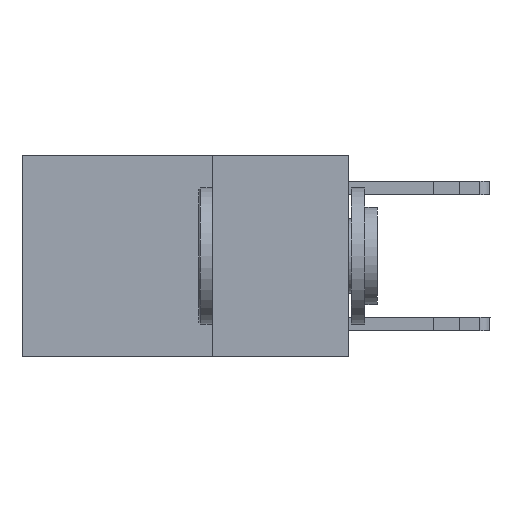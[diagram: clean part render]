
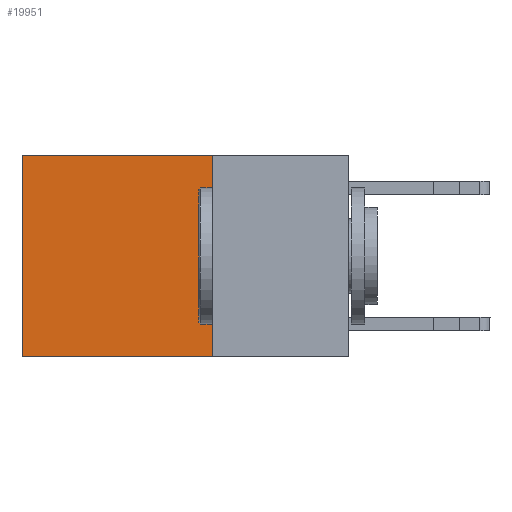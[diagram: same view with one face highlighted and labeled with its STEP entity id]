
A CAD part, left-side view. The second image highlights one B-rep face of the part: STEP entity #19951.
In plain terms, the highlighted planar face has unit normal (-1, 0, 0).
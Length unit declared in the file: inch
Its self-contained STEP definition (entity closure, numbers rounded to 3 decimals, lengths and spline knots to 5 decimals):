
#849 = VERTEX_POINT ( 'NONE', #15176 ) ;
#2041 = VERTEX_POINT ( 'NONE', #2257 ) ;
#2257 = CARTESIAN_POINT ( 'NONE',  ( 0.2625, 0.25, -0.37 ) ) ;
#2558 = EDGE_LOOP ( 'NONE', ( #5270, #16723, #10378, #8038 ) ) ;
#3212 = DIRECTION ( 'NONE',  ( 0., 0., -1. ) ) ;
#3309 = DIRECTION ( 'NONE',  ( 1., 0., 0. ) ) ;
#3355 = CARTESIAN_POINT ( 'NONE',  ( 0.2625, 0.25, 0. ) ) ;
#4119 = PLANE ( 'NONE',  #19130 ) ;
#4580 = EDGE_CURVE ( 'NONE', #13474, #21646, #9042, .T. ) ;
#5270 = ORIENTED_EDGE ( 'NONE', *, *, #4580, .T. ) ;
#5322 = CARTESIAN_POINT ( 'NONE',  ( 0.2625, 0.6, -0.37 ) ) ;
#5961 = CARTESIAN_POINT ( 'NONE',  ( 0.2625, 0.6, 0. ) ) ;
#8038 = ORIENTED_EDGE ( 'NONE', *, *, #8169, .T. ) ;
#8169 = EDGE_CURVE ( 'NONE', #849, #13474, #14391, .T. ) ;
#8604 = VECTOR ( 'NONE', #12992, 39.37008 ) ;
#9042 = LINE ( 'NONE', #13243, #8604 ) ;
#10378 = ORIENTED_EDGE ( 'NONE', *, *, #12121, .F. ) ;
#12121 = EDGE_CURVE ( 'NONE', #849, #2041, #20429, .T. ) ;
#12138 = EDGE_CURVE ( 'NONE', #2041, #21646, #20265, .T. ) ;
#12992 = DIRECTION ( 'NONE',  ( 0., 0., -1. ) ) ;
#13243 = CARTESIAN_POINT ( 'NONE',  ( 0.2625, 0.6, 0. ) ) ;
#13474 = VERTEX_POINT ( 'NONE', #5961 ) ;
#14140 = VECTOR ( 'NONE', #16469, 39.37008 ) ;
#14391 = LINE ( 'NONE', #17383, #14140 ) ;
#14678 = DIRECTION ( 'NONE',  ( 0., 1., 0. ) ) ;
#15176 = CARTESIAN_POINT ( 'NONE',  ( 0.2625, 0.25, 0. ) ) ;
#15285 = DIRECTION ( 'NONE',  ( 0., 0., -1. ) ) ;
#15394 = CARTESIAN_POINT ( 'NONE',  ( 0.2625, 0.25, 0. ) ) ;
#16171 = CARTESIAN_POINT ( 'NONE',  ( 0.2625, 0.25, -0.37 ) ) ;
#16469 = DIRECTION ( 'NONE',  ( 0., 1., 0. ) ) ;
#16723 = ORIENTED_EDGE ( 'NONE', *, *, #12138, .F. ) ;
#17383 = CARTESIAN_POINT ( 'NONE',  ( 0.2625, 0.25, 0. ) ) ;
#19045 = FACE_OUTER_BOUND ( 'NONE', #2558, .T. ) ;
#19130 = AXIS2_PLACEMENT_3D ( 'NONE', #3355, #3309, #3212 ) ;
#19951 = ADVANCED_FACE ( 'NONE', ( #19045 ), #4119, .F. ) ;
#20251 = VECTOR ( 'NONE', #14678, 39.37008 ) ;
#20265 = LINE ( 'NONE', #16171, #20251 ) ;
#20323 = VECTOR ( 'NONE', #15285, 39.37008 ) ;
#20429 = LINE ( 'NONE', #15394, #20323 ) ;
#21646 = VERTEX_POINT ( 'NONE', #5322 ) ;
